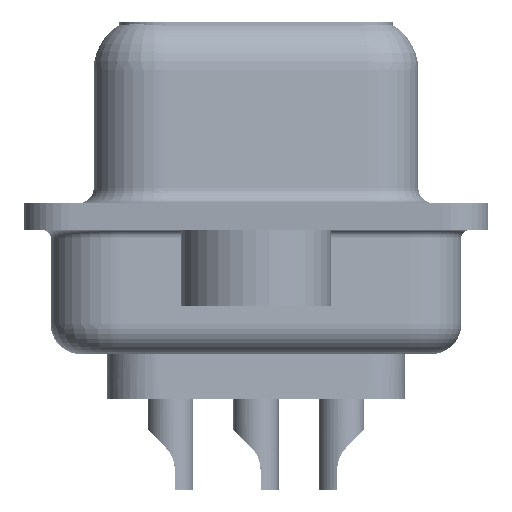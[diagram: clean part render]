
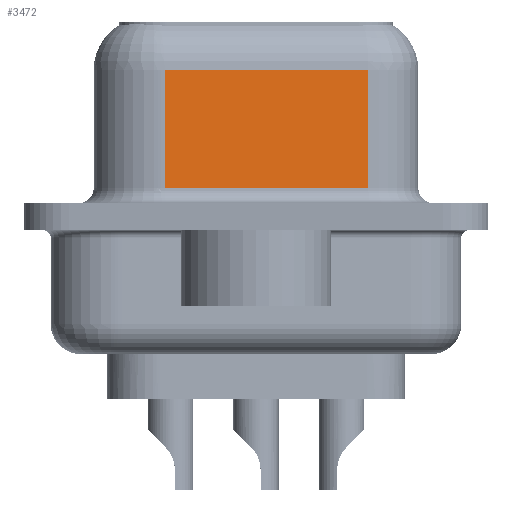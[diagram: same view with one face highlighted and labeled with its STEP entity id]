
A CAD part, left-side view. The second image highlights one B-rep face of the part: STEP entity #3472.
In plain terms, the highlighted planar face has unit normal (-0.985, -0.174, 0).
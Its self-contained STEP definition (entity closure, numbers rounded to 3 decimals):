
#3 = LINE ( 'NONE', #26498, #26554 ) ;
#1074 = EDGE_LOOP ( 'NONE', ( #34260, #7450, #13601, #31877 ) ) ;
#3181 = CARTESIAN_POINT ( 'NONE',  ( 5.621, -3.722, 0.95 ) ) ;
#3472 = ADVANCED_FACE ( 'NONE', ( #19543 ), #14267, .F. ) ;
#4376 = DIRECTION ( 'NONE',  ( -0.174, 0.985, 0. ) ) ;
#7286 = CARTESIAN_POINT ( 'NONE',  ( 5.621, -3.722, 4.85 ) ) ;
#7450 = ORIENTED_EDGE ( 'NONE', *, *, #26248, .T. ) ;
#8735 = EDGE_CURVE ( 'NONE', #25644, #20610, #33380, .T. ) ;
#13601 = ORIENTED_EDGE ( 'NONE', *, *, #15414, .T. ) ;
#14267 = PLANE ( 'NONE',  #34927 ) ;
#15414 = EDGE_CURVE ( 'NONE', #33957, #25644, #17840, .T. ) ;
#15523 = VECTOR ( 'NONE', #35189, 1000. ) ;
#17188 = DIRECTION ( 'NONE',  ( -0.174, 0.985, 0. ) ) ;
#17840 = LINE ( 'NONE', #29732, #15523 ) ;
#18436 = CARTESIAN_POINT ( 'NONE',  ( 4.43, 3.028, 4.85 ) ) ;
#18566 = DIRECTION ( 'NONE',  ( 0.174, -0.985, 0. ) ) ;
#19543 = FACE_OUTER_BOUND ( 'NONE', #1074, .T. ) ;
#20610 = VERTEX_POINT ( 'NONE', #20682 ) ;
#20682 = CARTESIAN_POINT ( 'NONE',  ( 5.621, -3.722, 0.95 ) ) ;
#22526 = VERTEX_POINT ( 'NONE', #26731 ) ;
#23360 = DIRECTION ( 'NONE',  ( 0., 0., -1. ) ) ;
#25644 = VERTEX_POINT ( 'NONE', #26425 ) ;
#25956 = DIRECTION ( 'NONE',  ( 0.985, 0.174, 0. ) ) ;
#26012 = VECTOR ( 'NONE', #18566, 1000. ) ;
#26248 = EDGE_CURVE ( 'NONE', #22526, #33957, #33981, .T. ) ;
#26425 = CARTESIAN_POINT ( 'NONE',  ( 4.43, 3.028, 0.95 ) ) ;
#26498 = CARTESIAN_POINT ( 'NONE',  ( 5.621, -3.722, 6.6 ) ) ;
#26554 = VECTOR ( 'NONE', #23360, 1000. ) ;
#26731 = CARTESIAN_POINT ( 'NONE',  ( 5.621, -3.722, 4.85 ) ) ;
#29732 = CARTESIAN_POINT ( 'NONE',  ( 4.43, 3.028, 6.6 ) ) ;
#31877 = ORIENTED_EDGE ( 'NONE', *, *, #8735, .T. ) ;
#32793 = VECTOR ( 'NONE', #4376, 1000. ) ;
#33380 = LINE ( 'NONE', #3181, #26012 ) ;
#33957 = VERTEX_POINT ( 'NONE', #18436 ) ;
#33981 = LINE ( 'NONE', #7286, #32793 ) ;
#34260 = ORIENTED_EDGE ( 'NONE', *, *, #34694, .F. ) ;
#34694 = EDGE_CURVE ( 'NONE', #22526, #20610, #3, .T. ) ;
#34911 = CARTESIAN_POINT ( 'NONE',  ( 5.621, -3.722, 6.6 ) ) ;
#34927 = AXIS2_PLACEMENT_3D ( 'NONE', #34911, #25956, #17188 ) ;
#35189 = DIRECTION ( 'NONE',  ( 0., 0., -1. ) ) ;
